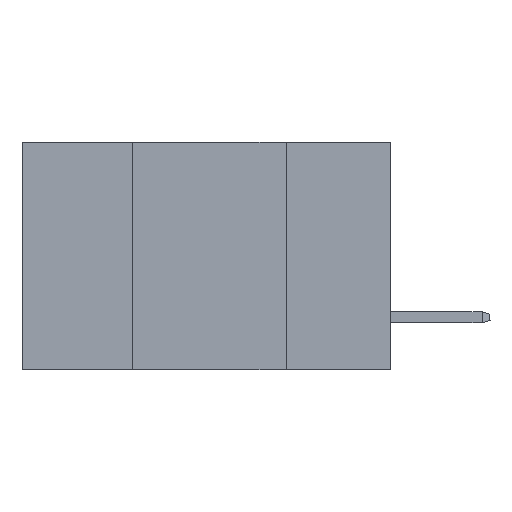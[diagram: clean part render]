
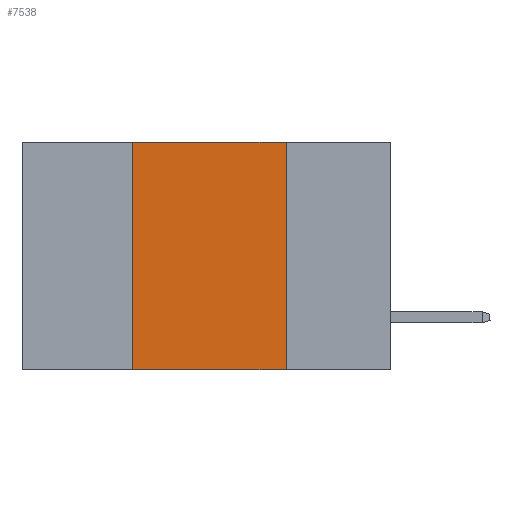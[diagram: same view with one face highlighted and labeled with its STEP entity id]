
A CAD part, left-side view. The second image highlights one B-rep face of the part: STEP entity #7538.
In plain terms, the highlighted planar face has unit normal (-1, 0, 0).
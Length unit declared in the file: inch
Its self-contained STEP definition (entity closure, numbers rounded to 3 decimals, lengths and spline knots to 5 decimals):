
#219 = VECTOR ( 'NONE', #3444, 39.37008 ) ;
#296 = VERTEX_POINT ( 'NONE', #8208 ) ;
#565 = VECTOR ( 'NONE', #9769, 39.37008 ) ;
#628 = EDGE_CURVE ( 'NONE', #2054, #751, #10925, .T. ) ;
#751 = VERTEX_POINT ( 'NONE', #6365 ) ;
#1523 = EDGE_CURVE ( 'NONE', #296, #1784, #3929, .T. ) ;
#1682 = EDGE_CURVE ( 'NONE', #2054, #296, #6123, .T. ) ;
#1688 = CARTESIAN_POINT ( 'NONE',  ( 0., 0.42, 0. ) ) ;
#1784 = VERTEX_POINT ( 'NONE', #3880 ) ;
#2054 = VERTEX_POINT ( 'NONE', #8179 ) ;
#2063 = AXIS2_PLACEMENT_3D ( 'NONE', #8788, #3653, #2868 ) ;
#2149 = PLANE ( 'NONE',  #2063 ) ;
#2868 = DIRECTION ( 'NONE',  ( 0., 0., -1. ) ) ;
#3027 = DIRECTION ( 'NONE',  ( 0., -1., 0. ) ) ;
#3145 = ORIENTED_EDGE ( 'NONE', *, *, #1523, .F. ) ;
#3444 = DIRECTION ( 'NONE',  ( 0., 0., 1. ) ) ;
#3641 = ORIENTED_EDGE ( 'NONE', *, *, #628, .T. ) ;
#3653 = DIRECTION ( 'NONE',  ( 1., 0., 0. ) ) ;
#3749 = CARTESIAN_POINT ( 'NONE',  ( 0., 0.17, 0. ) ) ;
#3880 = CARTESIAN_POINT ( 'NONE',  ( 0., 0.17, 0. ) ) ;
#3929 = LINE ( 'NONE', #4000, #10383 ) ;
#4000 = CARTESIAN_POINT ( 'NONE',  ( 0., 0.6, 0. ) ) ;
#4479 = VECTOR ( 'NONE', #10615, 39.37008 ) ;
#4540 = ORIENTED_EDGE ( 'NONE', *, *, #1682, .F. ) ;
#5244 = LINE ( 'NONE', #3749, #565 ) ;
#5486 = EDGE_LOOP ( 'NONE', ( #7963, #3145, #4540, #3641 ) ) ;
#5579 = EDGE_CURVE ( 'NONE', #1784, #751, #5244, .T. ) ;
#6123 = LINE ( 'NONE', #1688, #219 ) ;
#6365 = CARTESIAN_POINT ( 'NONE',  ( 0., 0.17, -0.37 ) ) ;
#7538 = ADVANCED_FACE ( 'NONE', ( #8364 ), #2149, .F. ) ;
#7963 = ORIENTED_EDGE ( 'NONE', *, *, #5579, .F. ) ;
#8179 = CARTESIAN_POINT ( 'NONE',  ( 0., 0.42, -0.37 ) ) ;
#8208 = CARTESIAN_POINT ( 'NONE',  ( 0., 0.42, 0. ) ) ;
#8364 = FACE_OUTER_BOUND ( 'NONE', #5486, .T. ) ;
#8788 = CARTESIAN_POINT ( 'NONE',  ( 0., 0.6, 0. ) ) ;
#9658 = CARTESIAN_POINT ( 'NONE',  ( 0., 0.6, -0.37 ) ) ;
#9769 = DIRECTION ( 'NONE',  ( 0., 0., -1. ) ) ;
#10383 = VECTOR ( 'NONE', #3027, 39.37008 ) ;
#10615 = DIRECTION ( 'NONE',  ( 0., -1., 0. ) ) ;
#10925 = LINE ( 'NONE', #9658, #4479 ) ;
